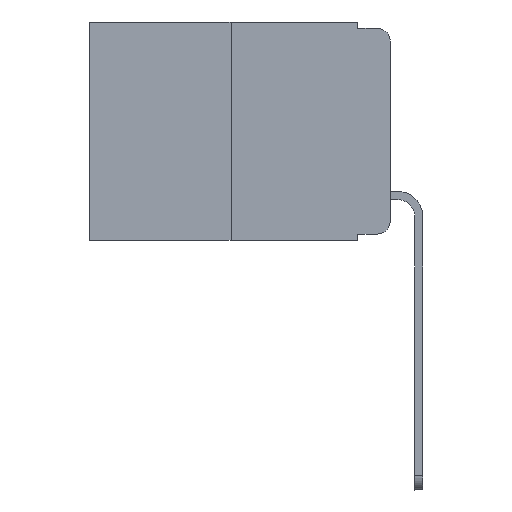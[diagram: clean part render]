
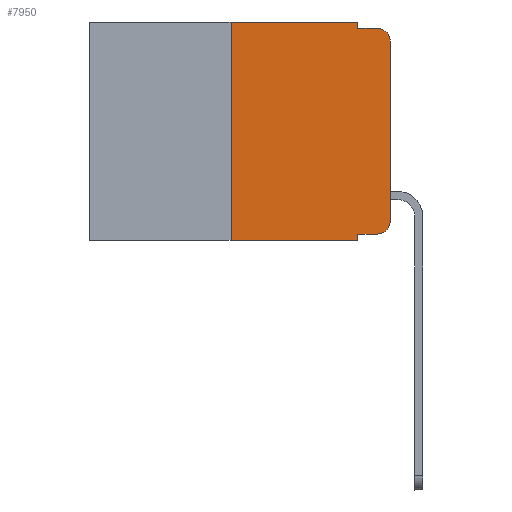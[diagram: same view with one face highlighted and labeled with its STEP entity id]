
A CAD part, left-side view. The second image highlights one B-rep face of the part: STEP entity #7950.
In plain terms, the highlighted planar face has unit normal (-1, 0, 0).
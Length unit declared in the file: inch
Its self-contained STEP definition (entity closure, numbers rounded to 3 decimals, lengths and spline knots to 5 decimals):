
#84 = CARTESIAN_POINT ( 'NONE',  ( 0., 0.051, -0.333 ) ) ;
#91 = LINE ( 'NONE', #12772, #10370 ) ;
#272 = LINE ( 'NONE', #11827, #13330 ) ;
#727 = VERTEX_POINT ( 'NONE', #12183 ) ;
#979 = DIRECTION ( 'NONE',  ( -1., 0., 0. ) ) ;
#1066 = LINE ( 'NONE', #10149, #6503 ) ;
#1230 = VECTOR ( 'NONE', #4681, 39.37008 ) ;
#1338 = DIRECTION ( 'NONE',  ( 0., 0., 1. ) ) ;
#1365 = CARTESIAN_POINT ( 'NONE',  ( 0., 0.051, 0. ) ) ;
#1416 = ORIENTED_EDGE ( 'NONE', *, *, #5395, .F. ) ;
#1452 = EDGE_CURVE ( 'NONE', #4102, #10607, #11581, .T. ) ;
#1749 = LINE ( 'NONE', #7521, #4109 ) ;
#2534 = LINE ( 'NONE', #10420, #6809 ) ;
#2893 = DIRECTION ( 'NONE',  ( 0., -1., 0. ) ) ;
#3142 = EDGE_LOOP ( 'NONE', ( #12677, #9790, #10154, #8088, #11608, #1416, #12397, #14790, #8074, #9566 ) ) ;
#3265 = DIRECTION ( 'NONE',  ( 0., 0., -1. ) ) ;
#3616 = LINE ( 'NONE', #1365, #11730 ) ;
#3867 = AXIS2_PLACEMENT_3D ( 'NONE', #8998, #979, #13746 ) ;
#3878 = FACE_OUTER_BOUND ( 'NONE', #3142, .T. ) ;
#4102 = VERTEX_POINT ( 'NONE', #11741 ) ;
#4109 = VECTOR ( 'NONE', #7735, 39.37008 ) ;
#4681 = DIRECTION ( 'NONE',  ( 0., -1., 0. ) ) ;
#4766 = DIRECTION ( 'NONE',  ( 0., -1., 0. ) ) ;
#4885 = CARTESIAN_POINT ( 'NONE',  ( 0., 0.051, -0.343 ) ) ;
#4931 = PLANE ( 'NONE',  #6515 ) ;
#5009 = DIRECTION ( 'NONE',  ( 0., 0., 1. ) ) ;
#5213 = CARTESIAN_POINT ( 'NONE',  ( 0., 0.25, -0.343 ) ) ;
#5395 = EDGE_CURVE ( 'NONE', #13803, #13111, #2534, .T. ) ;
#5781 = EDGE_CURVE ( 'NONE', #14054, #7774, #11433, .T. ) ;
#6124 = LINE ( 'NONE', #14298, #10317 ) ;
#6195 = VERTEX_POINT ( 'NONE', #11409 ) ;
#6503 = VECTOR ( 'NONE', #14726, 39.37008 ) ;
#6515 = AXIS2_PLACEMENT_3D ( 'NONE', #10692, #9636, #10919 ) ;
#6642 = CARTESIAN_POINT ( 'NONE',  ( 0., 0.02, -0.333 ) ) ;
#6809 = VECTOR ( 'NONE', #1338, 39.37008 ) ;
#7228 = CARTESIAN_POINT ( 'NONE',  ( 0., 0., -0.03 ) ) ;
#7521 = CARTESIAN_POINT ( 'NONE',  ( 0., 0.051, 0. ) ) ;
#7735 = DIRECTION ( 'NONE',  ( 0., 0., -1. ) ) ;
#7774 = VERTEX_POINT ( 'NONE', #10020 ) ;
#7950 = ADVANCED_FACE ( 'NONE', ( #3878 ), #4931, .F. ) ;
#8074 = ORIENTED_EDGE ( 'NONE', *, *, #1452, .T. ) ;
#8088 = ORIENTED_EDGE ( 'NONE', *, *, #9968, .F. ) ;
#8184 = DIRECTION ( 'NONE',  ( 0., 0., -1. ) ) ;
#8233 = EDGE_CURVE ( 'NONE', #13111, #727, #91, .T. ) ;
#8365 = CARTESIAN_POINT ( 'NONE',  ( 0., 0.051, -0.01 ) ) ;
#8583 = EDGE_CURVE ( 'NONE', #4102, #11712, #1749, .T. ) ;
#8693 = EDGE_CURVE ( 'NONE', #10607, #6195, #10332, .T. ) ;
#8998 = CARTESIAN_POINT ( 'NONE',  ( 0., 0.02, -0.313 ) ) ;
#9240 = EDGE_CURVE ( 'NONE', #9306, #7774, #6124, .T. ) ;
#9306 = VERTEX_POINT ( 'NONE', #8365 ) ;
#9566 = ORIENTED_EDGE ( 'NONE', *, *, #8693, .T. ) ;
#9636 = DIRECTION ( 'NONE',  ( 1., 0., 0. ) ) ;
#9790 = ORIENTED_EDGE ( 'NONE', *, *, #5781, .T. ) ;
#9968 = EDGE_CURVE ( 'NONE', #727, #9306, #3616, .T. ) ;
#10020 = CARTESIAN_POINT ( 'NONE',  ( 0., 0.02, -0.01 ) ) ;
#10149 = CARTESIAN_POINT ( 'NONE',  ( 0., 0.473, -0.343 ) ) ;
#10154 = ORIENTED_EDGE ( 'NONE', *, *, #9240, .F. ) ;
#10317 = VECTOR ( 'NONE', #2893, 39.37008 ) ;
#10332 = CIRCLE ( 'NONE', #3867, 0.02 ) ;
#10370 = VECTOR ( 'NONE', #4766, 39.37008 ) ;
#10420 = CARTESIAN_POINT ( 'NONE',  ( 0., 0.25, 0. ) ) ;
#10607 = VERTEX_POINT ( 'NONE', #6642 ) ;
#10692 = CARTESIAN_POINT ( 'NONE',  ( 0., 0.473, 0. ) ) ;
#10716 = AXIS2_PLACEMENT_3D ( 'NONE', #13545, #11298, #3265 ) ;
#10919 = DIRECTION ( 'NONE',  ( 0., 0., -1. ) ) ;
#11298 = DIRECTION ( 'NONE',  ( -1., 0., 0. ) ) ;
#11409 = CARTESIAN_POINT ( 'NONE',  ( 0., 0., -0.313 ) ) ;
#11433 = CIRCLE ( 'NONE', #10716, 0.02 ) ;
#11581 = LINE ( 'NONE', #84, #1230 ) ;
#11608 = ORIENTED_EDGE ( 'NONE', *, *, #8233, .F. ) ;
#11712 = VERTEX_POINT ( 'NONE', #4885 ) ;
#11730 = VECTOR ( 'NONE', #8184, 39.37008 ) ;
#11741 = CARTESIAN_POINT ( 'NONE',  ( 0., 0.051, -0.333 ) ) ;
#11827 = CARTESIAN_POINT ( 'NONE',  ( 0., 0., 0. ) ) ;
#12031 = EDGE_CURVE ( 'NONE', #6195, #14054, #272, .T. ) ;
#12183 = CARTESIAN_POINT ( 'NONE',  ( 0., 0.051, 0. ) ) ;
#12397 = ORIENTED_EDGE ( 'NONE', *, *, #13918, .T. ) ;
#12677 = ORIENTED_EDGE ( 'NONE', *, *, #12031, .T. ) ;
#12772 = CARTESIAN_POINT ( 'NONE',  ( 0., 0.473, 0. ) ) ;
#13111 = VERTEX_POINT ( 'NONE', #13411 ) ;
#13330 = VECTOR ( 'NONE', #5009, 39.37008 ) ;
#13411 = CARTESIAN_POINT ( 'NONE',  ( 0., 0.25, 0. ) ) ;
#13545 = CARTESIAN_POINT ( 'NONE',  ( 0., 0.02, -0.03 ) ) ;
#13746 = DIRECTION ( 'NONE',  ( 0., 0., -1. ) ) ;
#13803 = VERTEX_POINT ( 'NONE', #5213 ) ;
#13918 = EDGE_CURVE ( 'NONE', #13803, #11712, #1066, .T. ) ;
#14054 = VERTEX_POINT ( 'NONE', #7228 ) ;
#14298 = CARTESIAN_POINT ( 'NONE',  ( 0., 0.051, -0.01 ) ) ;
#14726 = DIRECTION ( 'NONE',  ( 0., -1., 0. ) ) ;
#14790 = ORIENTED_EDGE ( 'NONE', *, *, #8583, .F. ) ;
